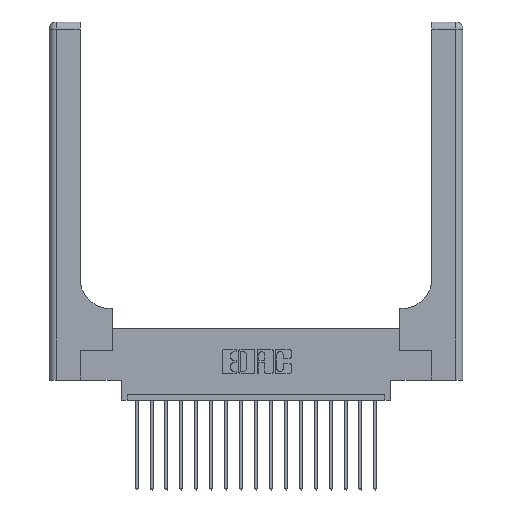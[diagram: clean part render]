
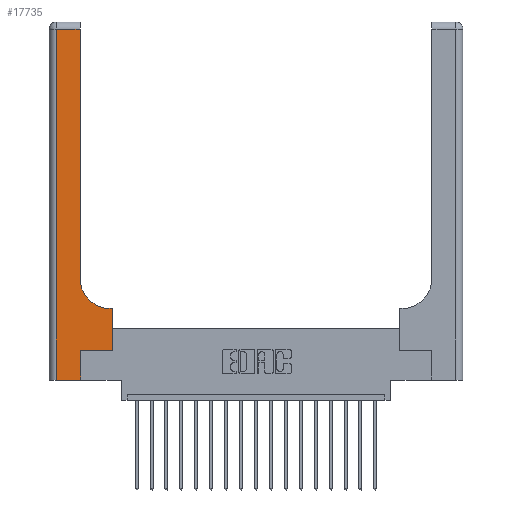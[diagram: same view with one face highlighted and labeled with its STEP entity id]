
A CAD part, top view. The second image highlights one B-rep face of the part: STEP entity #17735.
In plain terms, the highlighted planar face has unit normal (0, 0, 1).
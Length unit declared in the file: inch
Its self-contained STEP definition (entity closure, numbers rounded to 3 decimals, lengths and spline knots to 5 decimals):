
#107 = LINE ( 'NONE', #3294, #11584 ) ;
#1109 = ORIENTED_EDGE ( 'NONE', *, *, #7221, .T. ) ;
#1354 = CARTESIAN_POINT ( 'NONE',  ( 0.265, 0.25, 0.37 ) ) ;
#1732 = VERTEX_POINT ( 'NONE', #13982 ) ;
#1840 = VECTOR ( 'NONE', #16551, 39.37008 ) ;
#2069 = CARTESIAN_POINT ( 'NONE',  ( 0.265, 0.25, 0.37 ) ) ;
#2770 = AXIS2_PLACEMENT_3D ( 'NONE', #11821, #5178, #19490 ) ;
#3011 = LINE ( 'NONE', #4301, #8099 ) ;
#3273 = CARTESIAN_POINT ( 'NONE',  ( 0.26, 3., 0.37 ) ) ;
#3294 = CARTESIAN_POINT ( 'NONE',  ( 0.265, 0., 0.37 ) ) ;
#4301 = CARTESIAN_POINT ( 'NONE',  ( 0., 0., 0.37 ) ) ;
#5161 = DIRECTION ( 'NONE',  ( 1., 0., 0. ) ) ;
#5178 = DIRECTION ( 'NONE',  ( 0., 0., -1. ) ) ;
#5349 = PLANE ( 'NONE',  #9136 ) ;
#5613 = LINE ( 'NONE', #11503, #12225 ) ;
#5699 = VERTEX_POINT ( 'NONE', #15792 ) ;
#5886 = CARTESIAN_POINT ( 'NONE',  ( 0.06, 3., 0.37 ) ) ;
#6111 = VERTEX_POINT ( 'NONE', #9495 ) ;
#7031 = EDGE_CURVE ( 'NONE', #11672, #1732, #5613, .T. ) ;
#7221 = EDGE_CURVE ( 'NONE', #6111, #5699, #3011, .T. ) ;
#7249 = DIRECTION ( 'NONE',  ( -1., 0., 0. ) ) ;
#8099 = VECTOR ( 'NONE', #9086, 39.37008 ) ;
#8283 = ORIENTED_EDGE ( 'NONE', *, *, #19048, .T. ) ;
#8443 = CARTESIAN_POINT ( 'NONE',  ( 0., 3., 0.37 ) ) ;
#8541 = FACE_OUTER_BOUND ( 'NONE', #16795, .T. ) ;
#9086 = DIRECTION ( 'NONE',  ( 1., 0., 0. ) ) ;
#9094 = DIRECTION ( 'NONE',  ( -1., 0., 0. ) ) ;
#9136 = AXIS2_PLACEMENT_3D ( 'NONE', #8443, #13034, #7249 ) ;
#9249 = ORIENTED_EDGE ( 'NONE', *, *, #13299, .T. ) ;
#9353 = DIRECTION ( 'NONE',  ( 0., 1., 0. ) ) ;
#9476 = ORIENTED_EDGE ( 'NONE', *, *, #13924, .T. ) ;
#9495 = CARTESIAN_POINT ( 'NONE',  ( 0.06, 0., 0.37 ) ) ;
#9903 = EDGE_CURVE ( 'NONE', #12563, #11672, #11063, .T. ) ;
#10306 = ORIENTED_EDGE ( 'NONE', *, *, #9903, .T. ) ;
#10678 = LINE ( 'NONE', #5886, #1840 ) ;
#11063 = LINE ( 'NONE', #2069, #18084 ) ;
#11503 = CARTESIAN_POINT ( 'NONE',  ( 0.528, 0.25, 0.37 ) ) ;
#11584 = VECTOR ( 'NONE', #18449, 39.37008 ) ;
#11672 = VERTEX_POINT ( 'NONE', #18176 ) ;
#11821 = CARTESIAN_POINT ( 'NONE',  ( 0.51, 0.85, 0.37 ) ) ;
#12225 = VECTOR ( 'NONE', #19366, 39.37008 ) ;
#12335 = ORIENTED_EDGE ( 'NONE', *, *, #18314, .T. ) ;
#12338 = VECTOR ( 'NONE', #9094, 39.37008 ) ;
#12563 = VERTEX_POINT ( 'NONE', #1354 ) ;
#12638 = ORIENTED_EDGE ( 'NONE', *, *, #18665, .T. ) ;
#12907 = VECTOR ( 'NONE', #9353, 39.37008 ) ;
#13034 = DIRECTION ( 'NONE',  ( 0., 0., -1. ) ) ;
#13299 = EDGE_CURVE ( 'NONE', #13950, #15557, #18976, .T. ) ;
#13332 = VERTEX_POINT ( 'NONE', #18878 ) ;
#13924 = EDGE_CURVE ( 'NONE', #5699, #12563, #107, .T. ) ;
#13950 = VERTEX_POINT ( 'NONE', #17050 ) ;
#13982 = CARTESIAN_POINT ( 'NONE',  ( 0.528, 0.6, 0.37 ) ) ;
#14063 = ORIENTED_EDGE ( 'NONE', *, *, #15507, .T. ) ;
#14498 = CARTESIAN_POINT ( 'NONE',  ( 0., 2.94, 0.37 ) ) ;
#15043 = VERTEX_POINT ( 'NONE', #15266 ) ;
#15061 = VECTOR ( 'NONE', #17682, 39.37008 ) ;
#15266 = CARTESIAN_POINT ( 'NONE',  ( 0.26, 0.85, 0.37 ) ) ;
#15287 = LINE ( 'NONE', #19660, #12338 ) ;
#15507 = EDGE_CURVE ( 'NONE', #15043, #13950, #16931, .T. ) ;
#15557 = VERTEX_POINT ( 'NONE', #15636 ) ;
#15636 = CARTESIAN_POINT ( 'NONE',  ( 0.06, 2.94, 0.37 ) ) ;
#15792 = CARTESIAN_POINT ( 'NONE',  ( 0.265, 0., 0.37 ) ) ;
#16551 = DIRECTION ( 'NONE',  ( 0., -1., 0. ) ) ;
#16795 = EDGE_LOOP ( 'NONE', ( #14063, #9249, #12638, #1109, #9476, #10306, #18829, #12335, #8283 ) ) ;
#16931 = LINE ( 'NONE', #3273, #12907 ) ;
#17050 = CARTESIAN_POINT ( 'NONE',  ( 0.26, 2.94, 0.37 ) ) ;
#17411 = CIRCLE ( 'NONE', #2770, 0.25 ) ;
#17682 = DIRECTION ( 'NONE',  ( -1., 0., 0. ) ) ;
#17735 = ADVANCED_FACE ( 'NONE', ( #8541 ), #5349, .F. ) ;
#18084 = VECTOR ( 'NONE', #5161, 39.37008 ) ;
#18176 = CARTESIAN_POINT ( 'NONE',  ( 0.528, 0.25, 0.37 ) ) ;
#18314 = EDGE_CURVE ( 'NONE', #1732, #13332, #15287, .T. ) ;
#18449 = DIRECTION ( 'NONE',  ( 0., 1., 0. ) ) ;
#18665 = EDGE_CURVE ( 'NONE', #15557, #6111, #10678, .T. ) ;
#18829 = ORIENTED_EDGE ( 'NONE', *, *, #7031, .T. ) ;
#18878 = CARTESIAN_POINT ( 'NONE',  ( 0.51, 0.6, 0.37 ) ) ;
#18976 = LINE ( 'NONE', #14498, #15061 ) ;
#19048 = EDGE_CURVE ( 'NONE', #13332, #15043, #17411, .T. ) ;
#19366 = DIRECTION ( 'NONE',  ( 0., 1., 0. ) ) ;
#19490 = DIRECTION ( 'NONE',  ( 1., 0., 0. ) ) ;
#19660 = CARTESIAN_POINT ( 'NONE',  ( 0.26, 0.6, 0.37 ) ) ;
